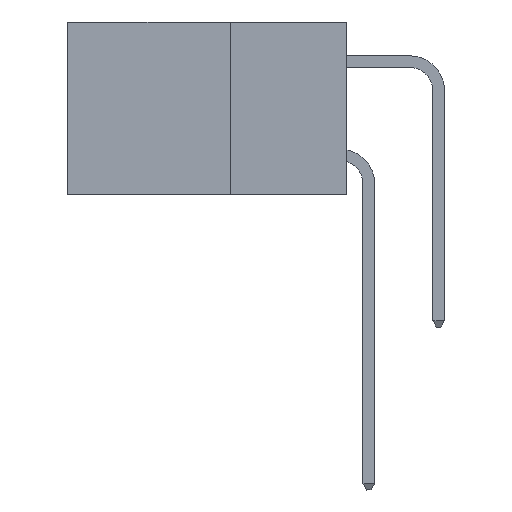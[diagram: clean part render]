
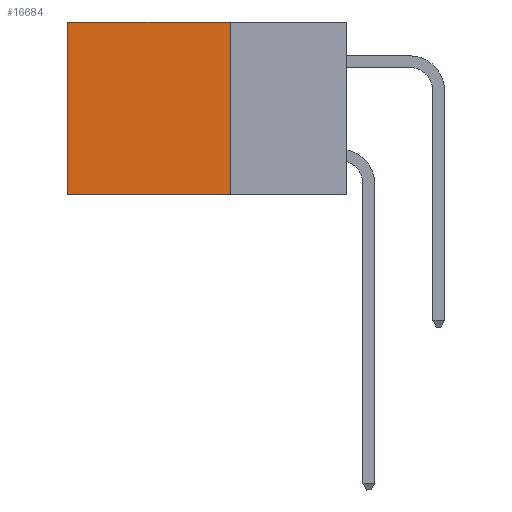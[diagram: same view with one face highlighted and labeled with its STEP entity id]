
A CAD part, left-side view. The second image highlights one B-rep face of the part: STEP entity #16684.
In plain terms, the highlighted planar face has unit normal (-1, 0, 0).
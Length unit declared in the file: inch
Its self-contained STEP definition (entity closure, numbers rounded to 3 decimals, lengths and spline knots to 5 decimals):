
#1638 = DIRECTION ( 'NONE',  ( 0., 1., 0. ) ) ;
#1697 = EDGE_CURVE ( 'NONE', #12859, #1962, #8924, .T. ) ;
#1962 = VERTEX_POINT ( 'NONE', #37231 ) ;
#4484 = VERTEX_POINT ( 'NONE', #30687 ) ;
#6447 = CARTESIAN_POINT ( 'NONE',  ( 0.2875, 0.25, 0. ) ) ;
#6959 = EDGE_LOOP ( 'NONE', ( #17242, #35613, #10916, #39581 ) ) ;
#8594 = EDGE_CURVE ( 'NONE', #21818, #12859, #18175, .T. ) ;
#8924 = LINE ( 'NONE', #42669, #35133 ) ;
#10916 = ORIENTED_EDGE ( 'NONE', *, *, #8594, .F. ) ;
#12304 = DIRECTION ( 'NONE',  ( 0., 1., 0. ) ) ;
#12859 = VERTEX_POINT ( 'NONE', #21540 ) ;
#12874 = VECTOR ( 'NONE', #16988, 39.37008 ) ;
#13498 = DIRECTION ( 'NONE',  ( 0., 0., -1. ) ) ;
#14037 = DIRECTION ( 'NONE',  ( 1., 0., 0. ) ) ;
#14453 = EDGE_CURVE ( 'NONE', #4484, #1962, #36415, .T. ) ;
#14488 = DIRECTION ( 'NONE',  ( 0., 0., -1. ) ) ;
#16586 = LINE ( 'NONE', #43280, #28320 ) ;
#16684 = ADVANCED_FACE ( 'NONE', ( #38541 ), #31358, .F. ) ;
#16988 = DIRECTION ( 'NONE',  ( 0., 0., -1. ) ) ;
#17242 = ORIENTED_EDGE ( 'NONE', *, *, #14453, .T. ) ;
#18175 = LINE ( 'NONE', #6447, #43364 ) ;
#21540 = CARTESIAN_POINT ( 'NONE',  ( 0.2875, 0.25, -0.37 ) ) ;
#21818 = VERTEX_POINT ( 'NONE', #35254 ) ;
#28320 = VECTOR ( 'NONE', #12304, 39.37008 ) ;
#29000 = CARTESIAN_POINT ( 'NONE',  ( 0.2875, 0.6, 0. ) ) ;
#30687 = CARTESIAN_POINT ( 'NONE',  ( 0.2875, 0.6, 0. ) ) ;
#31358 = PLANE ( 'NONE',  #34084 ) ;
#34084 = AXIS2_PLACEMENT_3D ( 'NONE', #34472, #14037, #14488 ) ;
#34472 = CARTESIAN_POINT ( 'NONE',  ( 0.2875, 0.25, 0. ) ) ;
#35133 = VECTOR ( 'NONE', #1638, 39.37008 ) ;
#35254 = CARTESIAN_POINT ( 'NONE',  ( 0.2875, 0.25, 0. ) ) ;
#35613 = ORIENTED_EDGE ( 'NONE', *, *, #1697, .F. ) ;
#36415 = LINE ( 'NONE', #29000, #12874 ) ;
#37231 = CARTESIAN_POINT ( 'NONE',  ( 0.2875, 0.6, -0.37 ) ) ;
#38541 = FACE_OUTER_BOUND ( 'NONE', #6959, .T. ) ;
#39165 = EDGE_CURVE ( 'NONE', #21818, #4484, #16586, .T. ) ;
#39581 = ORIENTED_EDGE ( 'NONE', *, *, #39165, .T. ) ;
#42669 = CARTESIAN_POINT ( 'NONE',  ( 0.2875, 0.25, -0.37 ) ) ;
#43280 = CARTESIAN_POINT ( 'NONE',  ( 0.2875, 0.25, 0. ) ) ;
#43364 = VECTOR ( 'NONE', #13498, 39.37008 ) ;
